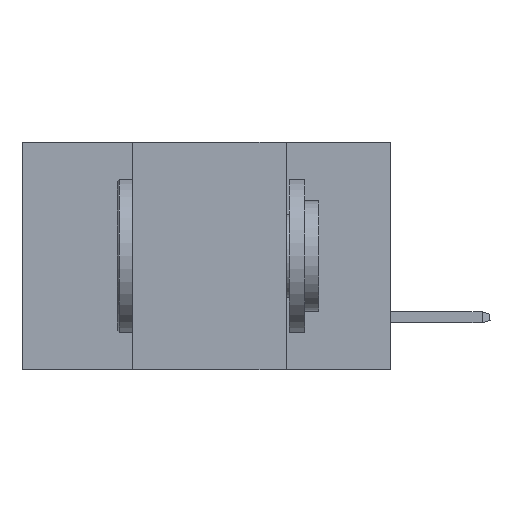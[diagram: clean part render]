
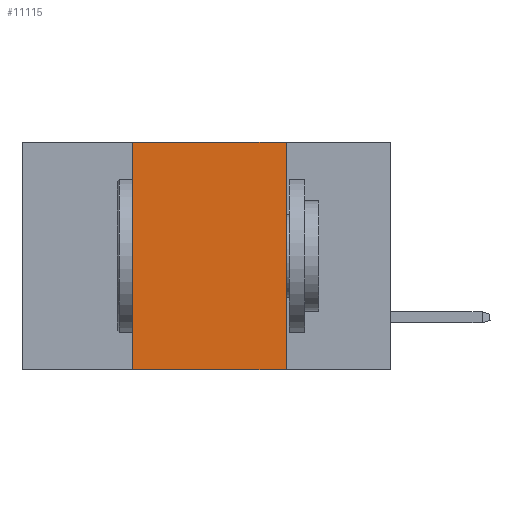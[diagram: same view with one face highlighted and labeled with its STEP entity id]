
A CAD part, left-side view. The second image highlights one B-rep face of the part: STEP entity #11115.
In plain terms, the highlighted planar face has unit normal (-1, 0, 0).
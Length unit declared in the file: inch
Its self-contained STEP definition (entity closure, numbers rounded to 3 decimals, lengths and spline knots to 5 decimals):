
#2856 = CARTESIAN_POINT ( 'NONE',  ( 0., 0.42, 0. ) ) ;
#2911 = CARTESIAN_POINT ( 'NONE',  ( 0., 0.6, 0. ) ) ;
#2993 = LINE ( 'NONE', #2911, #8008 ) ;
#4354 = EDGE_CURVE ( 'NONE', #26401, #26704, #22408, .T. ) ;
#5045 = EDGE_CURVE ( 'NONE', #22896, #26704, #18026, .T. ) ;
#5631 = DIRECTION ( 'NONE',  ( 1., 0., 0. ) ) ;
#5983 = CARTESIAN_POINT ( 'NONE',  ( 0., 0.6, 0. ) ) ;
#6723 = CARTESIAN_POINT ( 'NONE',  ( 0., 0.42, -0.37 ) ) ;
#7210 = CARTESIAN_POINT ( 'NONE',  ( 0., 0.17, -0.37 ) ) ;
#8008 = VECTOR ( 'NONE', #18110, 39.37008 ) ;
#8782 = CARTESIAN_POINT ( 'NONE',  ( 0., 0.17, 0. ) ) ;
#9154 = EDGE_CURVE ( 'NONE', #22896, #17124, #12820, .T. ) ;
#9181 = ORIENTED_EDGE ( 'NONE', *, *, #9154, .F. ) ;
#10513 = CARTESIAN_POINT ( 'NONE',  ( 0., 0.6, -0.37 ) ) ;
#11115 = ADVANCED_FACE ( 'NONE', ( #17349 ), #18739, .F. ) ;
#11734 = DIRECTION ( 'NONE',  ( 0., 0., 1. ) ) ;
#12368 = VECTOR ( 'NONE', #27514, 39.37008 ) ;
#12463 = AXIS2_PLACEMENT_3D ( 'NONE', #5983, #5631, #16972 ) ;
#12820 = LINE ( 'NONE', #2856, #24798 ) ;
#13733 = DIRECTION ( 'NONE',  ( 0., 0., -1. ) ) ;
#16972 = DIRECTION ( 'NONE',  ( 0., 0., -1. ) ) ;
#17124 = VERTEX_POINT ( 'NONE', #21979 ) ;
#17349 = FACE_OUTER_BOUND ( 'NONE', #25379, .T. ) ;
#18026 = LINE ( 'NONE', #10513, #12368 ) ;
#18110 = DIRECTION ( 'NONE',  ( 0., -1., 0. ) ) ;
#18739 = PLANE ( 'NONE',  #12463 ) ;
#18833 = ORIENTED_EDGE ( 'NONE', *, *, #5045, .T. ) ;
#18903 = EDGE_CURVE ( 'NONE', #17124, #26401, #2993, .T. ) ;
#20329 = ORIENTED_EDGE ( 'NONE', *, *, #18903, .F. ) ;
#21979 = CARTESIAN_POINT ( 'NONE',  ( 0., 0.42, 0. ) ) ;
#22408 = LINE ( 'NONE', #24240, #26709 ) ;
#22896 = VERTEX_POINT ( 'NONE', #6723 ) ;
#24240 = CARTESIAN_POINT ( 'NONE',  ( 0., 0.17, 0. ) ) ;
#24798 = VECTOR ( 'NONE', #11734, 39.37008 ) ;
#25379 = EDGE_LOOP ( 'NONE', ( #26482, #20329, #9181, #18833 ) ) ;
#26401 = VERTEX_POINT ( 'NONE', #8782 ) ;
#26482 = ORIENTED_EDGE ( 'NONE', *, *, #4354, .F. ) ;
#26704 = VERTEX_POINT ( 'NONE', #7210 ) ;
#26709 = VECTOR ( 'NONE', #13733, 39.37008 ) ;
#27514 = DIRECTION ( 'NONE',  ( 0., -1., 0. ) ) ;
